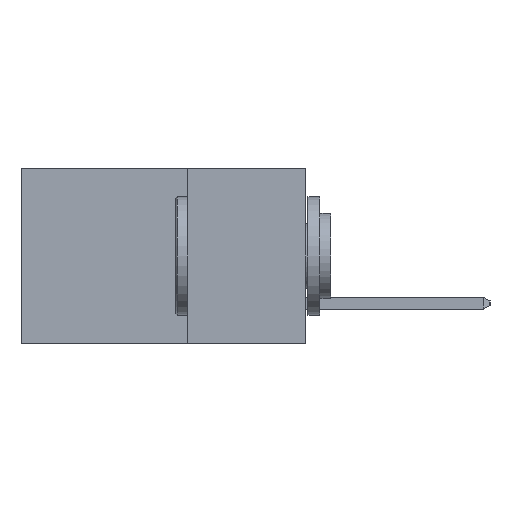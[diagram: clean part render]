
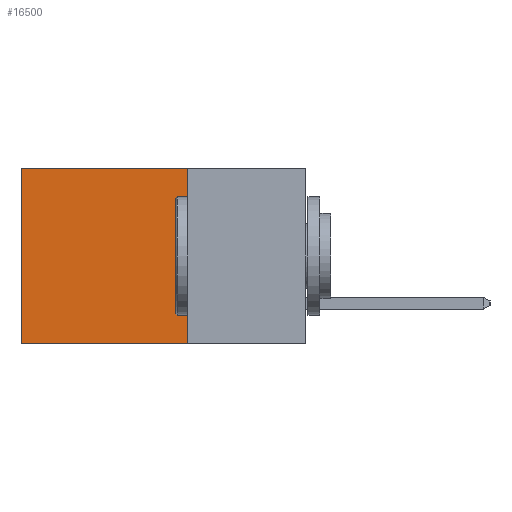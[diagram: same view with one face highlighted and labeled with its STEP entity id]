
A CAD part, left-side view. The second image highlights one B-rep face of the part: STEP entity #16500.
In plain terms, the highlighted planar face has unit normal (-1, 0, 0).
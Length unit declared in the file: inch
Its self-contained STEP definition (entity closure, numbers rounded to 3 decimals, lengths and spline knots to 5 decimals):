
#229 = VECTOR ( 'NONE', #18316, 39.37008 ) ;
#1033 = AXIS2_PLACEMENT_3D ( 'NONE', #17946, #4380, #16326 ) ;
#1075 = CARTESIAN_POINT ( 'NONE',  ( 0.298, 0.25, 0. ) ) ;
#1690 = EDGE_CURVE ( 'NONE', #10897, #10010, #14385, .T. ) ;
#2626 = PLANE ( 'NONE',  #1033 ) ;
#2913 = ORIENTED_EDGE ( 'NONE', *, *, #1690, .T. ) ;
#3636 = ORIENTED_EDGE ( 'NONE', *, *, #21168, .T. ) ;
#4380 = DIRECTION ( 'NONE',  ( 1., 0., 0. ) ) ;
#5287 = DIRECTION ( 'NONE',  ( 0., 1., 0. ) ) ;
#6542 = CARTESIAN_POINT ( 'NONE',  ( 0.298, 0.6, -0.37 ) ) ;
#7910 = EDGE_CURVE ( 'NONE', #21272, #11008, #19061, .T. ) ;
#10010 = VERTEX_POINT ( 'NONE', #19443 ) ;
#10768 = DIRECTION ( 'NONE',  ( 0., 1., 0. ) ) ;
#10897 = VERTEX_POINT ( 'NONE', #1075 ) ;
#10966 = CARTESIAN_POINT ( 'NONE',  ( 0.298, 0.25, -0.37 ) ) ;
#11008 = VERTEX_POINT ( 'NONE', #6542 ) ;
#12202 = CARTESIAN_POINT ( 'NONE',  ( 0.298, 0.25, -0.37 ) ) ;
#12362 = ORIENTED_EDGE ( 'NONE', *, *, #7910, .F. ) ;
#13545 = EDGE_LOOP ( 'NONE', ( #3636, #12362, #19574, #2913 ) ) ;
#13890 = LINE ( 'NONE', #19932, #229 ) ;
#14385 = LINE ( 'NONE', #16026, #18912 ) ;
#14548 = VECTOR ( 'NONE', #10768, 39.37008 ) ;
#14978 = LINE ( 'NONE', #15363, #18959 ) ;
#15181 = FACE_OUTER_BOUND ( 'NONE', #13545, .T. ) ;
#15363 = CARTESIAN_POINT ( 'NONE',  ( 0.298, 0.6, 0. ) ) ;
#16026 = CARTESIAN_POINT ( 'NONE',  ( 0.298, 0.25, 0. ) ) ;
#16326 = DIRECTION ( 'NONE',  ( 0., 0., -1. ) ) ;
#16500 = ADVANCED_FACE ( 'NONE', ( #15181 ), #2626, .F. ) ;
#17946 = CARTESIAN_POINT ( 'NONE',  ( 0.298, 0.25, 0. ) ) ;
#18316 = DIRECTION ( 'NONE',  ( 0., 0., -1. ) ) ;
#18912 = VECTOR ( 'NONE', #5287, 39.37008 ) ;
#18959 = VECTOR ( 'NONE', #22065, 39.37008 ) ;
#19061 = LINE ( 'NONE', #10966, #14548 ) ;
#19443 = CARTESIAN_POINT ( 'NONE',  ( 0.298, 0.6, 0. ) ) ;
#19574 = ORIENTED_EDGE ( 'NONE', *, *, #21624, .F. ) ;
#19932 = CARTESIAN_POINT ( 'NONE',  ( 0.298, 0.25, 0. ) ) ;
#21168 = EDGE_CURVE ( 'NONE', #10010, #11008, #14978, .T. ) ;
#21272 = VERTEX_POINT ( 'NONE', #12202 ) ;
#21624 = EDGE_CURVE ( 'NONE', #10897, #21272, #13890, .T. ) ;
#22065 = DIRECTION ( 'NONE',  ( 0., 0., -1. ) ) ;
